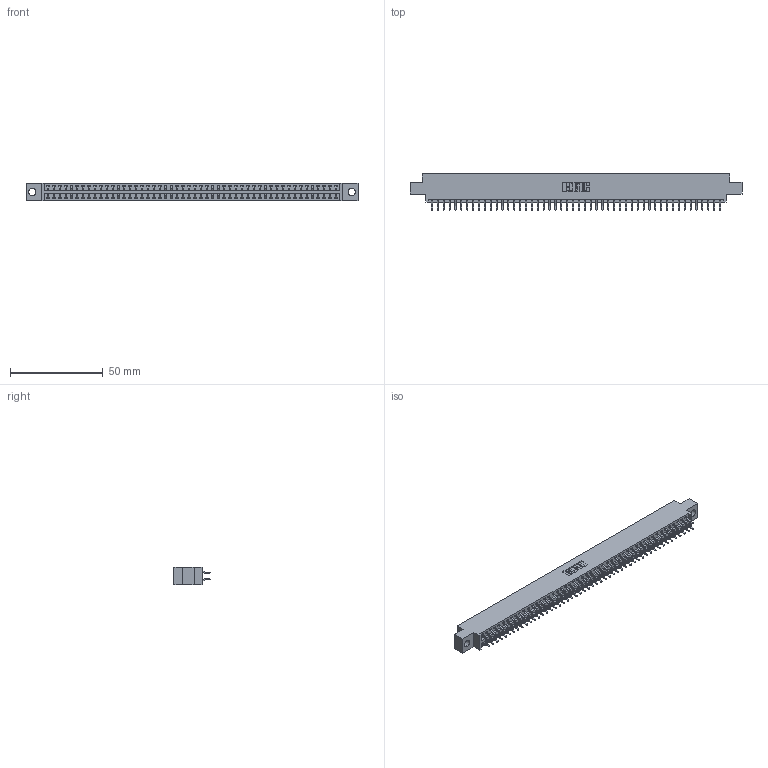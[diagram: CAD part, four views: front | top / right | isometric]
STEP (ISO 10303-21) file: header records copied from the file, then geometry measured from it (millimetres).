
FILE_DESCRIPTION (( 'STEP AP203' ), '1' );
FILE_NAME ('346-100-556-804.STEP', '2022-05-26T21:14:17', ( '' ), ( '' ), 'SwSTEP 2.0', 'SolidWorks 2020', '' );
FILE_SCHEMA (( 'CONFIG_CONTROL_DESIGN' ));
Length unit declared in the file: inch
Products named in the file (3): 346-100-556-804; 346 Part_0.170 Offset - 0.156 Dia-TH; 345-292-001_556 Tail
Assembly tree (101 placements, depth 2):
  346-100-556-804
    346 Part_0.170 Offset - 0.156 Dia-TH
    345-292-001_556 Tail  x100
Bounding box: 179.32 x 19.57 x 9.4 mm (x, y, z)
Volume: 17283.9 mm3; surface area: 23818.3 mm2
Topology: 101 solids, 101 shells, 5940 faces, 17677 edges, 11650 vertices
Faces by surface type: plane 3994, cylinder 1946
Entity records: 32325 total; most frequent: CARTESIAN_POINT 5338, ORIENTED_EDGE 5258, DIRECTION 4741, EDGE_CURVE 2629, LINE 2289, VECTOR 2289, VERTEX_POINT 1750, AXIS2_PLACEMENT_3D 1226
